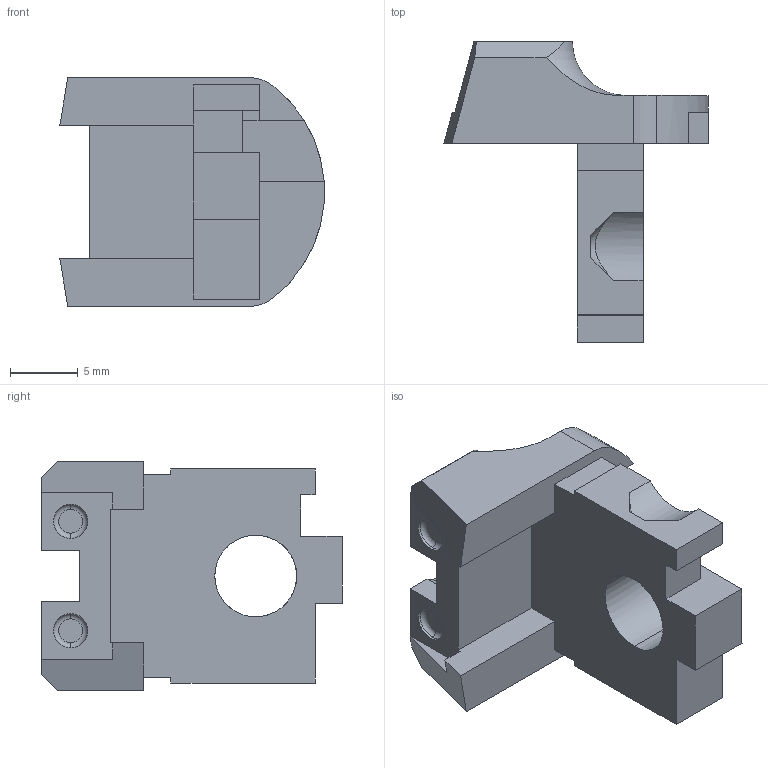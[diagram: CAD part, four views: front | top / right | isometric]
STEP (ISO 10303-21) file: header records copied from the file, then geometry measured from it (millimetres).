
FILE_DESCRIPTION (( 'STEP AP214' ), '1' );
FILE_NAME ('Rear Sight.step', '2014-07-30T19:46:36', ( 'WarFairy' ), ( '' ), 'SwSTEP 2.0', 'SolidWorks 2013', '' );
FILE_SCHEMA (( 'AUTOMOTIVE_DESIGN' ));
Length unit declared in the file: millimetre
Products named in the file (1): Rear Sight
Bounding box: 19.57 x 22.24 x 16.94 mm (x, y, z)
Volume: 1916.1 mm3; surface area: 1713 mm2
Topology: 1 solids, 1 shells, 75 faces, 208 edges, 136 vertices
Faces by surface type: plane 56, cylinder 12, torus 6, cone 1
Entity records: 2567 total; most frequent: CARTESIAN_POINT 477, ORIENTED_EDGE 416, DIRECTION 393, EDGE_CURVE 208, VECTOR 161, LINE 161, VERTEX_POINT 136, AXIS2_PLACEMENT_3D 116
